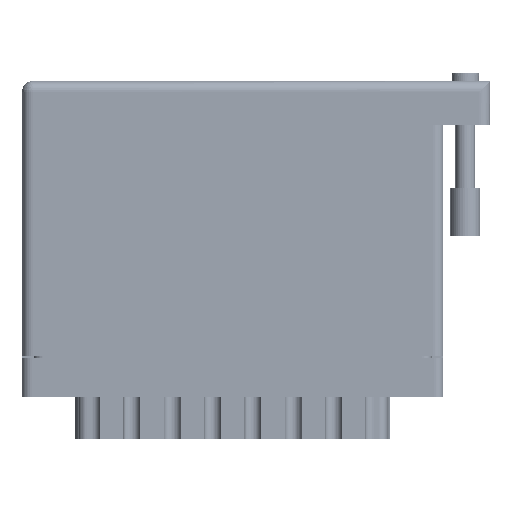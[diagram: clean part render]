
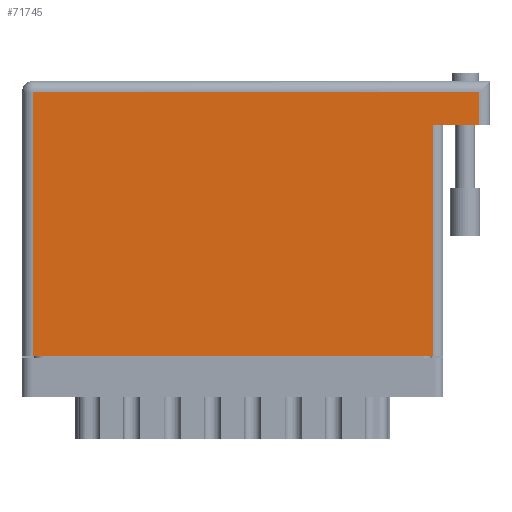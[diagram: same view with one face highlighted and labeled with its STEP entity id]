
A CAD part, front view. The second image highlights one B-rep face of the part: STEP entity #71745.
In plain terms, the highlighted face is planar.
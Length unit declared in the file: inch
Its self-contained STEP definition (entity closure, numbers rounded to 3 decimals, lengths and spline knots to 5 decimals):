
#1054 = AXIS2_PLACEMENT_3D ( 'NONE', #22150, #51263, #68787 ) ;
#3992 = VERTEX_POINT ( 'NONE', #32842 ) ;
#4011 = DIRECTION ( 'NONE',  ( 1., 0., 0. ) ) ;
#5093 = CARTESIAN_POINT ( 'NONE',  ( 0., 1.705, 0. ) ) ;
#5705 = VERTEX_POINT ( 'NONE', #55203 ) ;
#5844 = EDGE_CURVE ( 'NONE', #12990, #17906, #47129, .T. ) ;
#7501 = EDGE_CURVE ( 'NONE', #41610, #33181, #11909, .T. ) ;
#11909 = LINE ( 'NONE', #14106, #25784 ) ;
#12990 = VERTEX_POINT ( 'NONE', #22081 ) ;
#13176 = LINE ( 'NONE', #16065, #41802 ) ;
#14106 = CARTESIAN_POINT ( 'NONE',  ( 0.07, 0., 0. ) ) ;
#15756 = CARTESIAN_POINT ( 'NONE',  ( 0.07, 1.705, 0. ) ) ;
#16065 = CARTESIAN_POINT ( 'NONE',  ( 0., 0., 0. ) ) ;
#17668 = ORIENTED_EDGE ( 'NONE', *, *, #7501, .T. ) ;
#17906 = VERTEX_POINT ( 'NONE', #24045 ) ;
#18219 = CARTESIAN_POINT ( 'NONE',  ( 2.648, 1.495, 0. ) ) ;
#19273 = ORIENTED_EDGE ( 'NONE', *, *, #30457, .T. ) ;
#21024 = DIRECTION ( 'NONE',  ( 0., 1., 0. ) ) ;
#22081 = CARTESIAN_POINT ( 'NONE',  ( 2.948, 1.495, 0. ) ) ;
#22150 = CARTESIAN_POINT ( 'NONE',  ( 0., 1.775, 0. ) ) ;
#24045 = CARTESIAN_POINT ( 'NONE',  ( 2.648, 1.495, 0. ) ) ;
#24931 = ORIENTED_EDGE ( 'NONE', *, *, #44476, .T. ) ;
#25486 = DIRECTION ( 'NONE',  ( 0., 1., 0. ) ) ;
#25784 = VECTOR ( 'NONE', #72587, 39.37008 ) ;
#27975 = EDGE_CURVE ( 'NONE', #33181, #5705, #13176, .T. ) ;
#30457 = EDGE_CURVE ( 'NONE', #3992, #41610, #67501, .T. ) ;
#32634 = EDGE_LOOP ( 'NONE', ( #47699, #67167, #32938, #24931, #19273, #17668 ) ) ;
#32842 = CARTESIAN_POINT ( 'NONE',  ( 2.948, 1.705, 0. ) ) ;
#32938 = ORIENTED_EDGE ( 'NONE', *, *, #5844, .F. ) ;
#33181 = VERTEX_POINT ( 'NONE', #59201 ) ;
#37587 = CARTESIAN_POINT ( 'NONE',  ( 2.948, 1.775, 0. ) ) ;
#37929 = VECTOR ( 'NONE', #43429, 39.37008 ) ;
#40075 = LINE ( 'NONE', #37587, #68669 ) ;
#41610 = VERTEX_POINT ( 'NONE', #15756 ) ;
#41802 = VECTOR ( 'NONE', #4011, 39.37008 ) ;
#43429 = DIRECTION ( 'NONE',  ( -1., 0., 0. ) ) ;
#44464 = VECTOR ( 'NONE', #69496, 39.37008 ) ;
#44476 = EDGE_CURVE ( 'NONE', #12990, #3992, #40075, .T. ) ;
#46341 = FACE_OUTER_BOUND ( 'NONE', #32634, .T. ) ;
#47129 = LINE ( 'NONE', #61955, #37929 ) ;
#47699 = ORIENTED_EDGE ( 'NONE', *, *, #27975, .T. ) ;
#51263 = DIRECTION ( 'NONE',  ( 0., 0., -1. ) ) ;
#55203 = CARTESIAN_POINT ( 'NONE',  ( 2.648, 0., 0. ) ) ;
#56051 = VECTOR ( 'NONE', #25486, 39.37008 ) ;
#56973 = PLANE ( 'NONE',  #1054 ) ;
#59201 = CARTESIAN_POINT ( 'NONE',  ( 0.07, 0., 0. ) ) ;
#61955 = CARTESIAN_POINT ( 'NONE',  ( 3.018, 1.495, 0. ) ) ;
#65779 = EDGE_CURVE ( 'NONE', #5705, #17906, #73483, .T. ) ;
#67167 = ORIENTED_EDGE ( 'NONE', *, *, #65779, .T. ) ;
#67501 = LINE ( 'NONE', #5093, #44464 ) ;
#68669 = VECTOR ( 'NONE', #21024, 39.37008 ) ;
#68787 = DIRECTION ( 'NONE',  ( -1., 0., 0. ) ) ;
#69496 = DIRECTION ( 'NONE',  ( -1., 0., 0. ) ) ;
#71745 = ADVANCED_FACE ( 'NONE', ( #46341 ), #56973, .F. ) ;
#72587 = DIRECTION ( 'NONE',  ( 0., -1., 0. ) ) ;
#73483 = LINE ( 'NONE', #18219, #56051 ) ;
